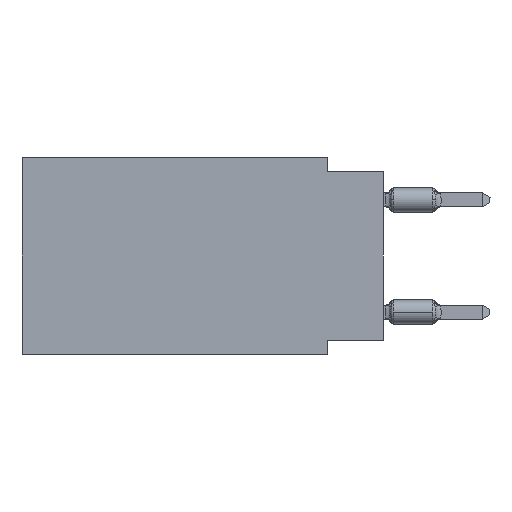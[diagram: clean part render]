
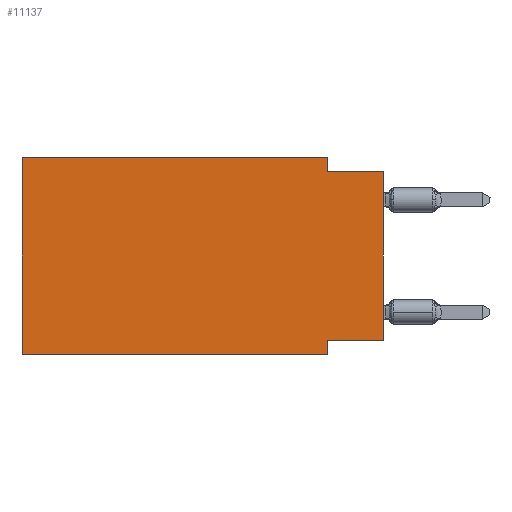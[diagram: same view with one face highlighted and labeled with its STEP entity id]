
A CAD part, left-side view. The second image highlights one B-rep face of the part: STEP entity #11137.
In plain terms, the highlighted planar face has unit normal (-1, 0, 0).
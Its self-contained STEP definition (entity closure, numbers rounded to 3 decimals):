
#160 = PLANE ( 'NONE',  #687 ) ;
#529 = ORIENTED_EDGE ( 'NONE', *, *, #9823, .F. ) ;
#687 = AXIS2_PLACEMENT_3D ( 'NONE', #28310, #10596, #35730 ) ;
#985 = VERTEX_POINT ( 'NONE', #45380 ) ;
#1154 = VECTOR ( 'NONE', #24228, 1000. ) ;
#1669 = VECTOR ( 'NONE', #14295, 1000. ) ;
#2985 = EDGE_CURVE ( 'NONE', #16824, #27000, #12477, .T. ) ;
#3189 = CARTESIAN_POINT ( 'NONE',  ( 0., 16.383, -8.89 ) ) ;
#3679 = VECTOR ( 'NONE', #28700, 1000. ) ;
#5320 = ORIENTED_EDGE ( 'NONE', *, *, #30895, .T. ) ;
#5406 = EDGE_CURVE ( 'NONE', #40036, #42123, #23321, .T. ) ;
#5507 = CARTESIAN_POINT ( 'NONE',  ( 0., 2.54, -8.89 ) ) ;
#6523 = CARTESIAN_POINT ( 'NONE',  ( 0., 0., -0.635 ) ) ;
#7284 = LINE ( 'NONE', #28937, #3679 ) ;
#7347 = FACE_OUTER_BOUND ( 'NONE', #37905, .T. ) ;
#7774 = ORIENTED_EDGE ( 'NONE', *, *, #40932, .F. ) ;
#9442 = VECTOR ( 'NONE', #14053, 1000. ) ;
#9823 = EDGE_CURVE ( 'NONE', #985, #30446, #19684, .T. ) ;
#10596 = DIRECTION ( 'NONE',  ( 1., 0., 0. ) ) ;
#11137 = ADVANCED_FACE ( 'NONE', ( #7347 ), #160, .F. ) ;
#12477 = LINE ( 'NONE', #5507, #34085 ) ;
#12669 = VECTOR ( 'NONE', #30631, 1000. ) ;
#14053 = DIRECTION ( 'NONE',  ( 0., 0., 1. ) ) ;
#14295 = DIRECTION ( 'NONE',  ( 0., 0., -1. ) ) ;
#15554 = EDGE_CURVE ( 'NONE', #43686, #42123, #7284, .T. ) ;
#15662 = LINE ( 'NONE', #25925, #31644 ) ;
#16472 = CARTESIAN_POINT ( 'NONE',  ( 0., 0., -0.635 ) ) ;
#16824 = VERTEX_POINT ( 'NONE', #17108 ) ;
#17108 = CARTESIAN_POINT ( 'NONE',  ( 0., 2.54, -8.255 ) ) ;
#17801 = LINE ( 'NONE', #31538, #1669 ) ;
#19684 = LINE ( 'NONE', #23661, #12669 ) ;
#21744 = CARTESIAN_POINT ( 'NONE',  ( 0., 16.383, 0. ) ) ;
#22393 = ORIENTED_EDGE ( 'NONE', *, *, #2985, .F. ) ;
#23321 = LINE ( 'NONE', #6523, #1154 ) ;
#23661 = CARTESIAN_POINT ( 'NONE',  ( 0., 16.383, 0. ) ) ;
#24228 = DIRECTION ( 'NONE',  ( 0., -1., 0. ) ) ;
#24399 = DIRECTION ( 'NONE',  ( 0., 1., 0. ) ) ;
#25684 = DIRECTION ( 'NONE',  ( 0., -1., 0. ) ) ;
#25925 = CARTESIAN_POINT ( 'NONE',  ( 0., 16.383, -8.89 ) ) ;
#26425 = CARTESIAN_POINT ( 'NONE',  ( 0., 2.54, 0. ) ) ;
#27000 = VERTEX_POINT ( 'NONE', #35812 ) ;
#28270 = LINE ( 'NONE', #21744, #9442 ) ;
#28310 = CARTESIAN_POINT ( 'NONE',  ( 0., 16.383, 0. ) ) ;
#28700 = DIRECTION ( 'NONE',  ( 0., 0., 1. ) ) ;
#28937 = CARTESIAN_POINT ( 'NONE',  ( 0., 0., 0. ) ) ;
#30446 = VERTEX_POINT ( 'NONE', #26425 ) ;
#30470 = LINE ( 'NONE', #35537, #36783 ) ;
#30631 = DIRECTION ( 'NONE',  ( 0., -1., 0. ) ) ;
#30895 = EDGE_CURVE ( 'NONE', #40605, #27000, #15662, .T. ) ;
#31538 = CARTESIAN_POINT ( 'NONE',  ( 0., 2.54, 0. ) ) ;
#31644 = VECTOR ( 'NONE', #25684, 1000. ) ;
#34085 = VECTOR ( 'NONE', #45035, 1000. ) ;
#34742 = EDGE_CURVE ( 'NONE', #40605, #985, #28270, .T. ) ;
#35537 = CARTESIAN_POINT ( 'NONE',  ( 0., 0., -8.255 ) ) ;
#35730 = DIRECTION ( 'NONE',  ( 0., 0., -1. ) ) ;
#35812 = CARTESIAN_POINT ( 'NONE',  ( 0., 2.54, -8.89 ) ) ;
#36783 = VECTOR ( 'NONE', #24399, 1000. ) ;
#37171 = ORIENTED_EDGE ( 'NONE', *, *, #5406, .F. ) ;
#37504 = CARTESIAN_POINT ( 'NONE',  ( 0., 2.54, -0.635 ) ) ;
#37905 = EDGE_LOOP ( 'NONE', ( #45633, #37171, #7774, #529, #38663, #5320, #22393, #41383 ) ) ;
#38663 = ORIENTED_EDGE ( 'NONE', *, *, #34742, .F. ) ;
#40036 = VERTEX_POINT ( 'NONE', #37504 ) ;
#40412 = CARTESIAN_POINT ( 'NONE',  ( 0., 0., -8.255 ) ) ;
#40605 = VERTEX_POINT ( 'NONE', #3189 ) ;
#40932 = EDGE_CURVE ( 'NONE', #30446, #40036, #17801, .T. ) ;
#41383 = ORIENTED_EDGE ( 'NONE', *, *, #45680, .F. ) ;
#42123 = VERTEX_POINT ( 'NONE', #16472 ) ;
#43686 = VERTEX_POINT ( 'NONE', #40412 ) ;
#45035 = DIRECTION ( 'NONE',  ( 0., 0., -1. ) ) ;
#45380 = CARTESIAN_POINT ( 'NONE',  ( 0., 16.383, 0. ) ) ;
#45633 = ORIENTED_EDGE ( 'NONE', *, *, #15554, .T. ) ;
#45680 = EDGE_CURVE ( 'NONE', #43686, #16824, #30470, .T. ) ;
